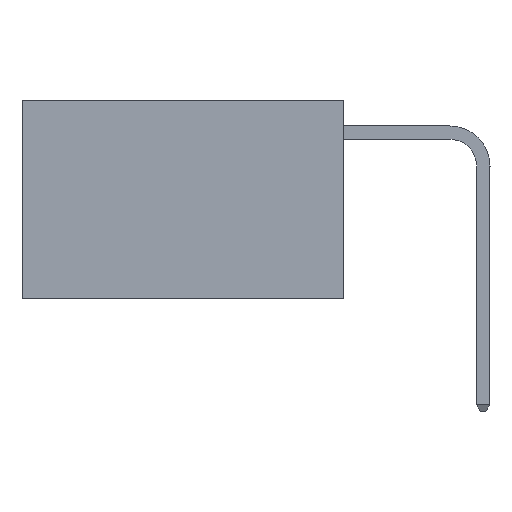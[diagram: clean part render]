
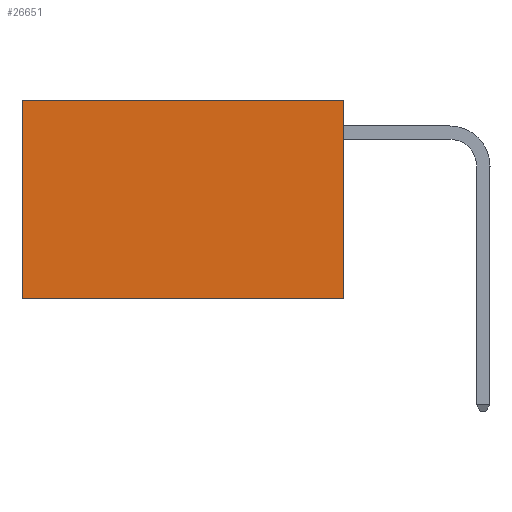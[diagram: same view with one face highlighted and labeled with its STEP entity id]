
A CAD part, left-side view. The second image highlights one B-rep face of the part: STEP entity #26651.
In plain terms, the highlighted planar face has unit normal (-1, 0, 0).
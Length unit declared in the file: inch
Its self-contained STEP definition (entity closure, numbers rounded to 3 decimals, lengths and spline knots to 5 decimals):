
#381 = DIRECTION ( 'NONE',  ( 0., 0., -1. ) ) ;
#409 = VECTOR ( 'NONE', #2244, 39.37008 ) ;
#1455 = VERTEX_POINT ( 'NONE', #4164 ) ;
#2244 = DIRECTION ( 'NONE',  ( 0., 0., -1. ) ) ;
#3378 = VECTOR ( 'NONE', #381, 39.37008 ) ;
#4164 = CARTESIAN_POINT ( 'NONE',  ( 0.2625, 0., -0.37 ) ) ;
#4175 = CARTESIAN_POINT ( 'NONE',  ( 0.2625, 0.6, 0. ) ) ;
#4635 = DIRECTION ( 'NONE',  ( 0., 0., -1. ) ) ;
#5443 = ORIENTED_EDGE ( 'NONE', *, *, #16769, .T. ) ;
#8218 = CARTESIAN_POINT ( 'NONE',  ( 0.2625, 0.6, -0.37 ) ) ;
#10319 = VERTEX_POINT ( 'NONE', #26543 ) ;
#10370 = ORIENTED_EDGE ( 'NONE', *, *, #21975, .T. ) ;
#10775 = ORIENTED_EDGE ( 'NONE', *, *, #25391, .F. ) ;
#11826 = CARTESIAN_POINT ( 'NONE',  ( 0.2625, 0., 0. ) ) ;
#12596 = EDGE_CURVE ( 'NONE', #10319, #1455, #19231, .T. ) ;
#13264 = PLANE ( 'NONE',  #25090 ) ;
#13958 = DIRECTION ( 'NONE',  ( 0., 1., 0. ) ) ;
#15182 = DIRECTION ( 'NONE',  ( 0., 1., 0. ) ) ;
#15384 = EDGE_LOOP ( 'NONE', ( #5443, #10775, #26066, #10370 ) ) ;
#15399 = CARTESIAN_POINT ( 'NONE',  ( 0.2625, 0., 0. ) ) ;
#16107 = VECTOR ( 'NONE', #15182, 39.37008 ) ;
#16687 = FACE_OUTER_BOUND ( 'NONE', #15384, .T. ) ;
#16769 = EDGE_CURVE ( 'NONE', #22283, #23958, #18369, .T. ) ;
#17529 = DIRECTION ( 'NONE',  ( 1., 0., 0. ) ) ;
#18102 = VECTOR ( 'NONE', #13958, 39.37008 ) ;
#18369 = LINE ( 'NONE', #21566, #409 ) ;
#19231 = LINE ( 'NONE', #26163, #3378 ) ;
#21566 = CARTESIAN_POINT ( 'NONE',  ( 0.2625, 0.6, 0. ) ) ;
#21743 = LINE ( 'NONE', #23555, #16107 ) ;
#21975 = EDGE_CURVE ( 'NONE', #10319, #22283, #23756, .T. ) ;
#22283 = VERTEX_POINT ( 'NONE', #4175 ) ;
#23555 = CARTESIAN_POINT ( 'NONE',  ( 0.2625, 0., -0.37 ) ) ;
#23756 = LINE ( 'NONE', #11826, #18102 ) ;
#23958 = VERTEX_POINT ( 'NONE', #8218 ) ;
#25090 = AXIS2_PLACEMENT_3D ( 'NONE', #15399, #17529, #4635 ) ;
#25391 = EDGE_CURVE ( 'NONE', #1455, #23958, #21743, .T. ) ;
#26066 = ORIENTED_EDGE ( 'NONE', *, *, #12596, .F. ) ;
#26163 = CARTESIAN_POINT ( 'NONE',  ( 0.2625, 0., 0. ) ) ;
#26543 = CARTESIAN_POINT ( 'NONE',  ( 0.2625, 0., 0. ) ) ;
#26651 = ADVANCED_FACE ( 'NONE', ( #16687 ), #13264, .F. ) ;
